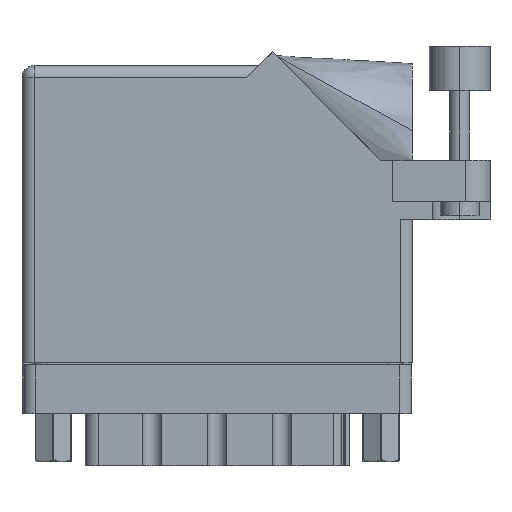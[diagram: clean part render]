
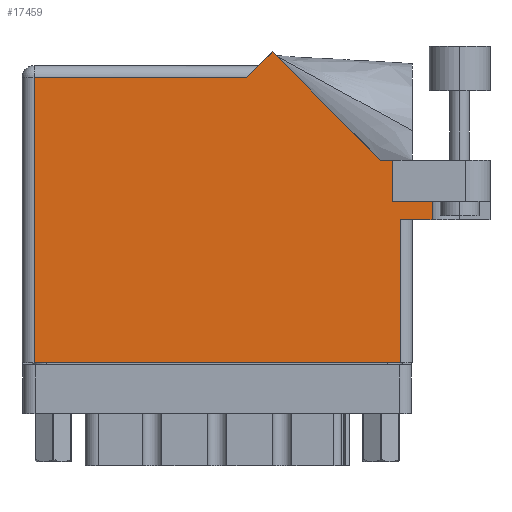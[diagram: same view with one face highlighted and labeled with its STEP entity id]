
A CAD part, front view. The second image highlights one B-rep face of the part: STEP entity #17459.
In plain terms, the highlighted face is planar.
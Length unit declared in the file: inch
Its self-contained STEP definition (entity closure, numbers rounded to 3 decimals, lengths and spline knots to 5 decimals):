
#1 = CARTESIAN_POINT ( 'NONE',  ( 0.062, 0., 0. ) ) ;
#1279 = LINE ( 'NONE', #23023, #38321 ) ;
#1702 = EDGE_CURVE ( 'NONE', #16399, #43060, #45435, .T. ) ;
#3535 = AXIS2_PLACEMENT_3D ( 'NONE', #11192, #26785, #15267 ) ;
#3801 = CARTESIAN_POINT ( 'NONE',  ( 2.1115, 0.737, 0. ) ) ;
#4458 = DIRECTION ( 'NONE',  ( -1., 0., 0. ) ) ;
#7036 = DIRECTION ( 'NONE',  ( 1., 0., 0. ) ) ;
#7217 = EDGE_LOOP ( 'NONE', ( #47503, #27623, #30715, #26857, #10798, #24792, #34967, #15929, #17293, #43820, #21703 ) ) ;
#7456 = VECTOR ( 'NONE', #20272, 39.37008 ) ;
#8277 = LINE ( 'NONE', #10026, #45317 ) ;
#9050 = LINE ( 'NONE', #43840, #45484 ) ;
#9328 = LINE ( 'NONE', #14324, #37877 ) ;
#10026 = CARTESIAN_POINT ( 'NONE',  ( 1.948, 0.737, 0. ) ) ;
#10216 = DIRECTION ( 'NONE',  ( -1., 0., 0. ) ) ;
#10798 = ORIENTED_EDGE ( 'NONE', *, *, #32435, .F. ) ;
#10981 = LINE ( 'NONE', #44577, #21345 ) ;
#11192 = CARTESIAN_POINT ( 'NONE',  ( 0., 1.53, 0. ) ) ;
#11806 = EDGE_CURVE ( 'NONE', #45810, #17415, #10981, .T. ) ;
#12456 = CARTESIAN_POINT ( 'NONE',  ( 0., 1.468, 0. ) ) ;
#13943 = DIRECTION ( 'NONE',  ( 0., 1., 0. ) ) ;
#14050 = EDGE_CURVE ( 'NONE', #41615, #36455, #41154, .T. ) ;
#14276 = EDGE_CURVE ( 'NONE', #31454, #48141, #8277, .T. ) ;
#14324 = CARTESIAN_POINT ( 'NONE',  ( 1.91, 0.831, 0. ) ) ;
#15188 = VECTOR ( 'NONE', #10216, 39.37008 ) ;
#15267 = DIRECTION ( 'NONE',  ( -1., 0., 0. ) ) ;
#15591 = LINE ( 'NONE', #30817, #22301 ) ;
#15929 = ORIENTED_EDGE ( 'NONE', *, *, #18177, .T. ) ;
#16399 = VERTEX_POINT ( 'NONE', #36735 ) ;
#16459 = CARTESIAN_POINT ( 'NONE',  ( 1.948, 0., 0. ) ) ;
#17293 = ORIENTED_EDGE ( 'NONE', *, *, #1702, .T. ) ;
#17415 = VERTEX_POINT ( 'NONE', #45990 ) ;
#17459 = ADVANCED_FACE ( 'NONE', ( #46914 ), #38514, .F. ) ;
#18177 = EDGE_CURVE ( 'NONE', #39721, #16399, #48767, .T. ) ;
#19887 = DIRECTION ( 'NONE',  ( -0.707, -0.707, 0. ) ) ;
#19924 = VECTOR ( 'NONE', #19887, 39.37008 ) ;
#20272 = DIRECTION ( 'NONE',  ( -0.707, 0.707, 0. ) ) ;
#21345 = VECTOR ( 'NONE', #28952, 39.37008 ) ;
#21471 = CARTESIAN_POINT ( 'NONE',  ( 2.1115, 0.831, 0. ) ) ;
#21703 = ORIENTED_EDGE ( 'NONE', *, *, #41129, .T. ) ;
#21852 = CARTESIAN_POINT ( 'NONE',  ( 1.91, 0.831, 0. ) ) ;
#22166 = EDGE_CURVE ( 'NONE', #43060, #49025, #38371, .T. ) ;
#22301 = VECTOR ( 'NONE', #26718, 39.37008 ) ;
#23023 = CARTESIAN_POINT ( 'NONE',  ( 0., 0., 0. ) ) ;
#23991 = CARTESIAN_POINT ( 'NONE',  ( 1.84442, 1.044, 0. ) ) ;
#24698 = CARTESIAN_POINT ( 'NONE',  ( 1.948, 0.737, 0. ) ) ;
#24792 = ORIENTED_EDGE ( 'NONE', *, *, #11806, .T. ) ;
#24987 = CARTESIAN_POINT ( 'NONE',  ( 2.1115, 1.16177, 0. ) ) ;
#25431 = EDGE_CURVE ( 'NONE', #17415, #39721, #43734, .T. ) ;
#26023 = DIRECTION ( 'NONE',  ( 1., 0., 0. ) ) ;
#26718 = DIRECTION ( 'NONE',  ( 0., -1., 0. ) ) ;
#26785 = DIRECTION ( 'NONE',  ( 0., 0., -1. ) ) ;
#26857 = ORIENTED_EDGE ( 'NONE', *, *, #14050, .F. ) ;
#27623 = ORIENTED_EDGE ( 'NONE', *, *, #14276, .T. ) ;
#28952 = DIRECTION ( 'NONE',  ( 0., 1., 0. ) ) ;
#29284 = EDGE_CURVE ( 'NONE', #48141, #36455, #9050, .T. ) ;
#30715 = ORIENTED_EDGE ( 'NONE', *, *, #29284, .T. ) ;
#30804 = VECTOR ( 'NONE', #40601, 39.37008 ) ;
#30817 = CARTESIAN_POINT ( 'NONE',  ( 0.062, 0., 0. ) ) ;
#31454 = VERTEX_POINT ( 'NONE', #16459 ) ;
#32435 = EDGE_CURVE ( 'NONE', #45810, #41615, #9328, .T. ) ;
#34967 = ORIENTED_EDGE ( 'NONE', *, *, #25431, .T. ) ;
#36455 = VERTEX_POINT ( 'NONE', #3801 ) ;
#36735 = CARTESIAN_POINT ( 'NONE',  ( 1.28771, 1.60071, 0. ) ) ;
#37877 = VECTOR ( 'NONE', #26023, 39.37008 ) ;
#38321 = VECTOR ( 'NONE', #7036, 39.37008 ) ;
#38371 = LINE ( 'NONE', #12456, #43843 ) ;
#38514 = PLANE ( 'NONE',  #3535 ) ;
#39583 = DIRECTION ( 'NONE',  ( 1., 0., 0. ) ) ;
#39721 = VERTEX_POINT ( 'NONE', #44985 ) ;
#40601 = DIRECTION ( 'NONE',  ( 0., -1., 0. ) ) ;
#41129 = EDGE_CURVE ( 'NONE', #49025, #44614, #15591, .T. ) ;
#41154 = LINE ( 'NONE', #24987, #30804 ) ;
#41615 = VERTEX_POINT ( 'NONE', #21471 ) ;
#43060 = VERTEX_POINT ( 'NONE', #43319 ) ;
#43319 = CARTESIAN_POINT ( 'NONE',  ( 1.155, 1.468, 0. ) ) ;
#43734 = LINE ( 'NONE', #48735, #15188 ) ;
#43820 = ORIENTED_EDGE ( 'NONE', *, *, #22166, .T. ) ;
#43840 = CARTESIAN_POINT ( 'NONE',  ( 2.01, 0.737, 0. ) ) ;
#43843 = VECTOR ( 'NONE', #4458, 39.37008 ) ;
#44577 = CARTESIAN_POINT ( 'NONE',  ( 1.91, 0.831, 0. ) ) ;
#44614 = VERTEX_POINT ( 'NONE', #1 ) ;
#44985 = CARTESIAN_POINT ( 'NONE',  ( 1.84442, 1.044, 0. ) ) ;
#45068 = EDGE_CURVE ( 'NONE', #44614, #31454, #1279, .T. ) ;
#45317 = VECTOR ( 'NONE', #13943, 39.37008 ) ;
#45319 = CARTESIAN_POINT ( 'NONE',  ( 0.062, 1.468, 0. ) ) ;
#45435 = LINE ( 'NONE', #46998, #19924 ) ;
#45484 = VECTOR ( 'NONE', #39583, 39.37008 ) ;
#45810 = VERTEX_POINT ( 'NONE', #21852 ) ;
#45990 = CARTESIAN_POINT ( 'NONE',  ( 1.91, 1.044, 0. ) ) ;
#46914 = FACE_OUTER_BOUND ( 'NONE', #7217, .T. ) ;
#46998 = CARTESIAN_POINT ( 'NONE',  ( 1.217, 1.53, 0. ) ) ;
#47503 = ORIENTED_EDGE ( 'NONE', *, *, #45068, .T. ) ;
#48141 = VERTEX_POINT ( 'NONE', #24698 ) ;
#48735 = CARTESIAN_POINT ( 'NONE',  ( 2.41, 1.044, 0. ) ) ;
#48767 = LINE ( 'NONE', #23991, #7456 ) ;
#49025 = VERTEX_POINT ( 'NONE', #45319 ) ;
